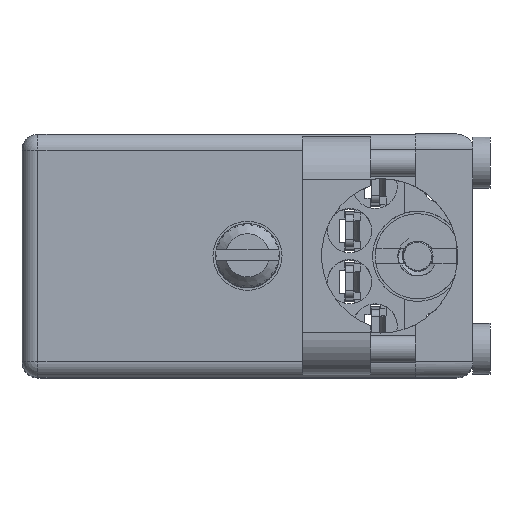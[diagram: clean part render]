
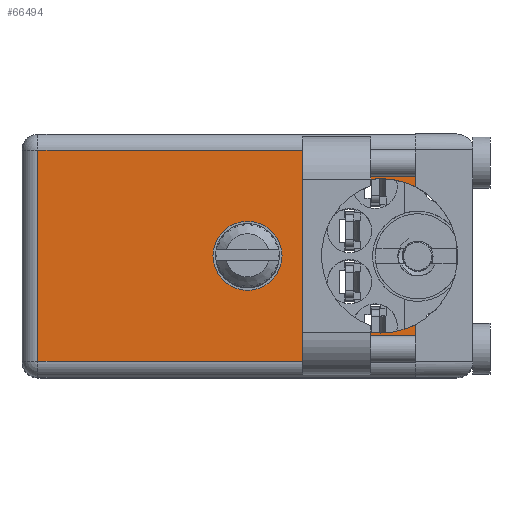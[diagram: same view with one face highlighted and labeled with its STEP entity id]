
A CAD part, top view. The second image highlights one B-rep face of the part: STEP entity #66494.
In plain terms, the highlighted face is planar.
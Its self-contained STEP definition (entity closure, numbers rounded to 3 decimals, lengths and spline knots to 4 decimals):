
#2402 = ORIENTED_EDGE ( 'NONE', *, *, #198549, .F. ) ;
#9424 = VECTOR ( 'NONE', #46540, 39.3701 ) ;
#10078 = ORIENTED_EDGE ( 'NONE', *, *, #86582, .T. ) ;
#10956 = DIRECTION ( 'NONE',  ( 0., 0., 1. ) ) ;
#13074 = CARTESIAN_POINT ( 'NONE',  ( 0.6625, 0.906, -0.3575 ) ) ;
#14345 = LINE ( 'NONE', #15342, #180801 ) ;
#15059 = DIRECTION ( 'NONE',  ( 0., 0., 1. ) ) ;
#15342 = CARTESIAN_POINT ( 'NONE',  ( 0., 0.906, -0.668 ) ) ;
#15986 = DIRECTION ( 'NONE',  ( 0., 0., 1. ) ) ;
#21787 = DIRECTION ( 'NONE',  ( 0., 0., 1. ) ) ;
#25352 = CARTESIAN_POINT ( 'NONE',  ( 1.155, 0.906, -0.047 ) ) ;
#25850 = DIRECTION ( 'NONE',  ( 0., 0., 1. ) ) ;
#26425 = AXIS2_PLACEMENT_3D ( 'NONE', #85124, #114360, #21787 ) ;
#26902 = VERTEX_POINT ( 'NONE', #138091 ) ;
#27451 = LINE ( 'NONE', #123008, #9424 ) ;
#28041 = AXIS2_PLACEMENT_3D ( 'NONE', #13074, #152856, #15059 ) ;
#39698 = EDGE_CURVE ( 'NONE', #107356, #73825, #14345, .T. ) ;
#46540 = DIRECTION ( 'NONE',  ( 0., 0., 1. ) ) ;
#46858 = EDGE_LOOP ( 'NONE', ( #60035, #183249 ) ) ;
#49758 = CIRCLE ( 'NONE', #104484, 0.227 ) ;
#50751 = ORIENTED_EDGE ( 'NONE', *, *, #39698, .T. ) ;
#52158 = CARTESIAN_POINT ( 'NONE',  ( 1.155, 0.906, -0.668 ) ) ;
#54713 = VERTEX_POINT ( 'NONE', #166999 ) ;
#56729 = EDGE_CURVE ( 'NONE', #62953, #99641, #174901, .T. ) ;
#58401 = EDGE_CURVE ( 'NONE', #164643, #112533, #117838, .T. ) ;
#58574 = EDGE_CURVE ( 'NONE', #26902, #164643, #146174, .T. ) ;
#60035 = ORIENTED_EDGE ( 'NONE', *, *, #92281, .F. ) ;
#61991 = ORIENTED_EDGE ( 'NONE', *, *, #58401, .F. ) ;
#62953 = VERTEX_POINT ( 'NONE', #78155 ) ;
#63099 = VECTOR ( 'NONE', #101828, 39.3701 ) ;
#65679 = ORIENTED_EDGE ( 'NONE', *, *, #80948, .F. ) ;
#66494 = ADVANCED_FACE ( 'NONE', ( #121883, #183228 ), #109770, .T. ) ;
#67758 = CARTESIAN_POINT ( 'NONE',  ( 1.053, 0.906, -0.5845 ) ) ;
#69067 = VECTOR ( 'NONE', #129013, 39.3701 ) ;
#72209 = AXIS2_PLACEMENT_3D ( 'NONE', #135935, #103767, #136907 ) ;
#73825 = VERTEX_POINT ( 'NONE', #99514 ) ;
#74565 = DIRECTION ( 'NONE',  ( 0., 1., 0. ) ) ;
#78155 = CARTESIAN_POINT ( 'NONE',  ( 1.155, 0.906, -0.5603 ) ) ;
#80948 = EDGE_CURVE ( 'NONE', #99641, #26902, #49758, .T. ) ;
#84738 = LINE ( 'NONE', #25352, #63099 ) ;
#85124 = CARTESIAN_POINT ( 'NONE',  ( 0.6625, 0.906, -0.3575 ) ) ;
#86232 = CARTESIAN_POINT ( 'NONE',  ( 1.053, 0.906, -0.3575 ) ) ;
#86582 = EDGE_CURVE ( 'NONE', #54713, #112533, #84738, .T. ) ;
#88134 = AXIS2_PLACEMENT_3D ( 'NONE', #154776, #139687, #15986 ) ;
#88364 = LINE ( 'NONE', #194025, #114911 ) ;
#92281 = EDGE_CURVE ( 'NONE', #153202, #196612, #162913, .T. ) ;
#93962 = CIRCLE ( 'NONE', #26425, 0.1015 ) ;
#99514 = CARTESIAN_POINT ( 'NONE',  ( 0.047, 0.906, -0.668 ) ) ;
#99641 = VERTEX_POINT ( 'NONE', #67758 ) ;
#101828 = DIRECTION ( 'NONE',  ( 1., 0., 0. ) ) ;
#103767 = DIRECTION ( 'NONE',  ( 0., 1., 0. ) ) ;
#104484 = AXIS2_PLACEMENT_3D ( 'NONE', #86232, #145635, #25850 ) ;
#106806 = DIRECTION ( 'NONE',  ( 0., 0., 1. ) ) ;
#107356 = VERTEX_POINT ( 'NONE', #52158 ) ;
#109770 = PLANE ( 'NONE',  #197150 ) ;
#112533 = VERTEX_POINT ( 'NONE', #194483 ) ;
#112923 = EDGE_CURVE ( 'NONE', #73825, #54713, #88364, .T. ) ;
#114360 = DIRECTION ( 'NONE',  ( 0., 1., 0. ) ) ;
#114911 = VECTOR ( 'NONE', #10956, 39.3701 ) ;
#117697 = ORIENTED_EDGE ( 'NONE', *, *, #112923, .T. ) ;
#117838 = LINE ( 'NONE', #193320, #69067 ) ;
#121883 = FACE_OUTER_BOUND ( 'NONE', #156168, .T. ) ;
#123008 = CARTESIAN_POINT ( 'NONE',  ( 1.155, 0.906, 0. ) ) ;
#127343 = CARTESIAN_POINT ( 'NONE',  ( 1.155, 0.906, -0.1547 ) ) ;
#129013 = DIRECTION ( 'NONE',  ( 0., 0., 1. ) ) ;
#135935 = CARTESIAN_POINT ( 'NONE',  ( 1.053, 0.906, -0.3575 ) ) ;
#136907 = DIRECTION ( 'NONE',  ( 0., 0., 1. ) ) ;
#138091 = CARTESIAN_POINT ( 'NONE',  ( 1.053, 0.906, -0.1305 ) ) ;
#139687 = DIRECTION ( 'NONE',  ( 0., 1., 0. ) ) ;
#145304 = ORIENTED_EDGE ( 'NONE', *, *, #56729, .F. ) ;
#145635 = DIRECTION ( 'NONE',  ( 0., 1., 0. ) ) ;
#146174 = CIRCLE ( 'NONE', #72209, 0.227 ) ;
#148671 = CARTESIAN_POINT ( 'NONE',  ( 0.6625, 0.906, -0.459 ) ) ;
#152856 = DIRECTION ( 'NONE',  ( 0., 1., 0. ) ) ;
#153202 = VERTEX_POINT ( 'NONE', #175525 ) ;
#154776 = CARTESIAN_POINT ( 'NONE',  ( 1.053, 0.906, -0.3575 ) ) ;
#156168 = EDGE_LOOP ( 'NONE', ( #2402, #50751, #117697, #10078, #61991, #175526, #65679, #145304 ) ) ;
#156769 = EDGE_CURVE ( 'NONE', #196612, #153202, #93962, .T. ) ;
#162913 = CIRCLE ( 'NONE', #28041, 0.1015 ) ;
#164643 = VERTEX_POINT ( 'NONE', #127343 ) ;
#166999 = CARTESIAN_POINT ( 'NONE',  ( 0.047, 0.906, -0.047 ) ) ;
#167210 = DIRECTION ( 'NONE',  ( -1., 0., 0. ) ) ;
#174901 = CIRCLE ( 'NONE', #88134, 0.227 ) ;
#175525 = CARTESIAN_POINT ( 'NONE',  ( 0.6625, 0.906, -0.256 ) ) ;
#175526 = ORIENTED_EDGE ( 'NONE', *, *, #58574, .F. ) ;
#180801 = VECTOR ( 'NONE', #167210, 39.3701 ) ;
#182222 = CARTESIAN_POINT ( 'NONE',  ( 0., 0.906, -0.715 ) ) ;
#183228 = FACE_BOUND ( 'NONE', #46858, .T. ) ;
#183249 = ORIENTED_EDGE ( 'NONE', *, *, #156769, .F. ) ;
#193320 = CARTESIAN_POINT ( 'NONE',  ( 1.155, 0.906, 0. ) ) ;
#194025 = CARTESIAN_POINT ( 'NONE',  ( 0.047, 0.906, -0.715 ) ) ;
#194483 = CARTESIAN_POINT ( 'NONE',  ( 1.155, 0.906, -0.047 ) ) ;
#196612 = VERTEX_POINT ( 'NONE', #148671 ) ;
#197150 = AXIS2_PLACEMENT_3D ( 'NONE', #182222, #74565, #106806 ) ;
#198549 = EDGE_CURVE ( 'NONE', #107356, #62953, #27451, .T. ) ;
